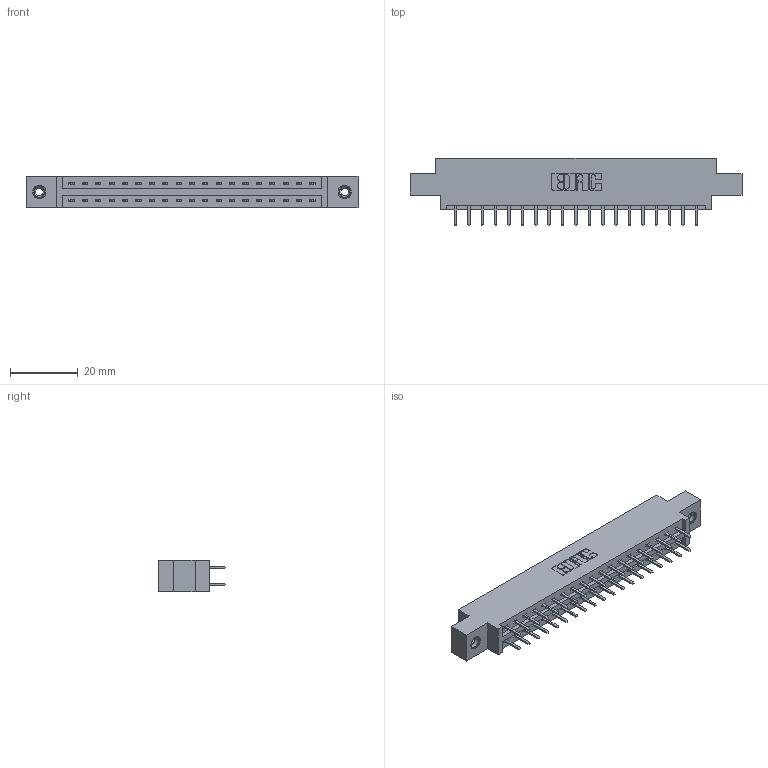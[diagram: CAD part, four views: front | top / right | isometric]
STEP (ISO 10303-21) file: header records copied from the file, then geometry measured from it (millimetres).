
FILE_DESCRIPTION (( 'STEP AP203' ), '1' );
FILE_NAME ('337-038-520-808.STEP', '2019-10-11T11:10:04', ( '' ), ( '' ), 'SwSTEP 2.0', 'SolidWorks 2016', '' );
FILE_SCHEMA (( 'CONFIG_CONTROL_DESIGN' ));
Length unit declared in the file: inch
Products named in the file (4): 337 Part_0.170 Offset - 0.156 Dia-TI; 337-038-520-808; 345-250-001_345-250-003-102; 345-292-001_345-293-120
Assembly tree (41 placements, depth 2):
  337-038-520-808
    337 Part_0.170 Offset - 0.156 Dia-TI
    345-292-001_345-293-120  x38
    345-250-001_345-250-003-102  x2
Bounding box: 98.3 x 20.02 x 9.4 mm (x, y, z)
Volume: 9912.5 mm3; surface area: 11066.8 mm2
Topology: 41 solids, 41 shells, 2382 faces, 6881 edges, 4478 vertices
Faces by surface type: plane 1626, cylinder 740, cone 12, torus 4
Entity records: 19138 total; most frequent: CARTESIAN_POINT 3237, ORIENTED_EDGE 3154, DIRECTION 2815, EDGE_CURVE 1577, VECTOR 1425, LINE 1425, VERTEX_POINT 1044, AXIS2_PLACEMENT_3D 695
